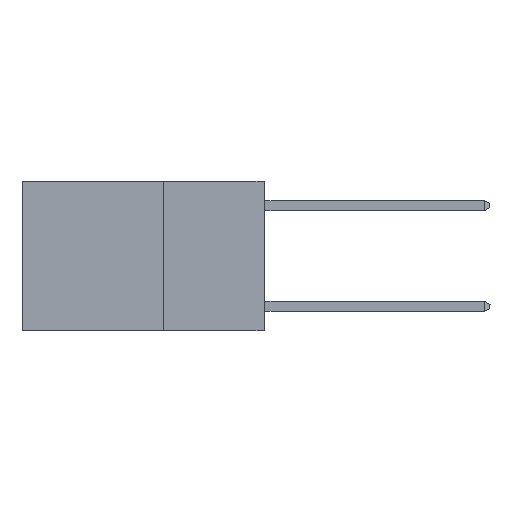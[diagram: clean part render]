
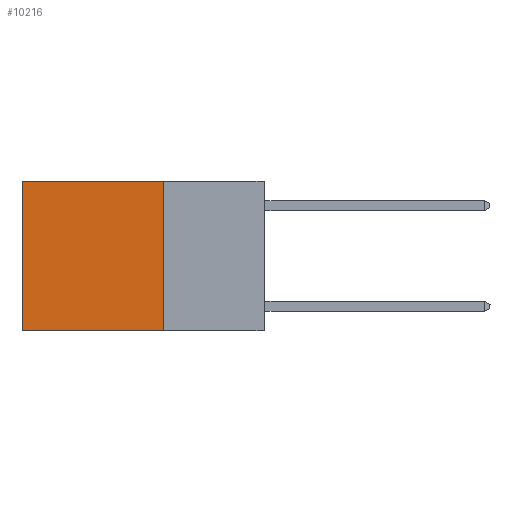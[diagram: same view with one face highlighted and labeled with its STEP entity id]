
A CAD part, left-side view. The second image highlights one B-rep face of the part: STEP entity #10216.
In plain terms, the highlighted planar face has unit normal (-1, 0, 0).
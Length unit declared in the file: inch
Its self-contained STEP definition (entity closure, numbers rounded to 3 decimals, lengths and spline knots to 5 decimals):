
#656 = ORIENTED_EDGE ( 'NONE', *, *, #10932, .F. ) ;
#2214 = VERTEX_POINT ( 'NONE', #17734 ) ;
#2512 = DIRECTION ( 'NONE',  ( 0., 0., -1. ) ) ;
#2942 = DIRECTION ( 'NONE',  ( 0., 1., 0. ) ) ;
#3549 = CARTESIAN_POINT ( 'NONE',  ( 0.2625, 0.25, -0.37 ) ) ;
#3988 = DIRECTION ( 'NONE',  ( 1., 0., 0. ) ) ;
#4421 = VECTOR ( 'NONE', #2942, 39.37008 ) ;
#4862 = CARTESIAN_POINT ( 'NONE',  ( 0.2625, 0.6, 0. ) ) ;
#5581 = VERTEX_POINT ( 'NONE', #16634 ) ;
#7238 = VECTOR ( 'NONE', #7830, 39.37008 ) ;
#7531 = EDGE_CURVE ( 'NONE', #10100, #2214, #18861, .T. ) ;
#7736 = VECTOR ( 'NONE', #15298, 39.37008 ) ;
#7830 = DIRECTION ( 'NONE',  ( 0., 0., -1. ) ) ;
#8007 = VECTOR ( 'NONE', #2512, 39.37008 ) ;
#8205 = ORIENTED_EDGE ( 'NONE', *, *, #7531, .T. ) ;
#8286 = EDGE_LOOP ( 'NONE', ( #8205, #10681, #656, #12132 ) ) ;
#8459 = LINE ( 'NONE', #11310, #8007 ) ;
#9810 = PLANE ( 'NONE',  #15654 ) ;
#10100 = VERTEX_POINT ( 'NONE', #12426 ) ;
#10216 = ADVANCED_FACE ( 'NONE', ( #12083 ), #9810, .F. ) ;
#10268 = CARTESIAN_POINT ( 'NONE',  ( 0.2625, 0.25, 0. ) ) ;
#10681 = ORIENTED_EDGE ( 'NONE', *, *, #12715, .F. ) ;
#10932 = EDGE_CURVE ( 'NONE', #14163, #5581, #8459, .T. ) ;
#11310 = CARTESIAN_POINT ( 'NONE',  ( 0.2625, 0.25, 0. ) ) ;
#11796 = CARTESIAN_POINT ( 'NONE',  ( 0.2625, 0.25, 0. ) ) ;
#12083 = FACE_OUTER_BOUND ( 'NONE', #8286, .T. ) ;
#12132 = ORIENTED_EDGE ( 'NONE', *, *, #14824, .T. ) ;
#12426 = CARTESIAN_POINT ( 'NONE',  ( 0.2625, 0.6, 0. ) ) ;
#12715 = EDGE_CURVE ( 'NONE', #5581, #2214, #15962, .T. ) ;
#12744 = CARTESIAN_POINT ( 'NONE',  ( 0.2625, 0.25, 0. ) ) ;
#14163 = VERTEX_POINT ( 'NONE', #11796 ) ;
#14248 = DIRECTION ( 'NONE',  ( 0., 0., -1. ) ) ;
#14824 = EDGE_CURVE ( 'NONE', #14163, #10100, #15671, .T. ) ;
#15298 = DIRECTION ( 'NONE',  ( 0., 1., 0. ) ) ;
#15654 = AXIS2_PLACEMENT_3D ( 'NONE', #12744, #3988, #14248 ) ;
#15671 = LINE ( 'NONE', #10268, #4421 ) ;
#15962 = LINE ( 'NONE', #3549, #7736 ) ;
#16634 = CARTESIAN_POINT ( 'NONE',  ( 0.2625, 0.25, -0.37 ) ) ;
#17734 = CARTESIAN_POINT ( 'NONE',  ( 0.2625, 0.6, -0.37 ) ) ;
#18861 = LINE ( 'NONE', #4862, #7238 ) ;
